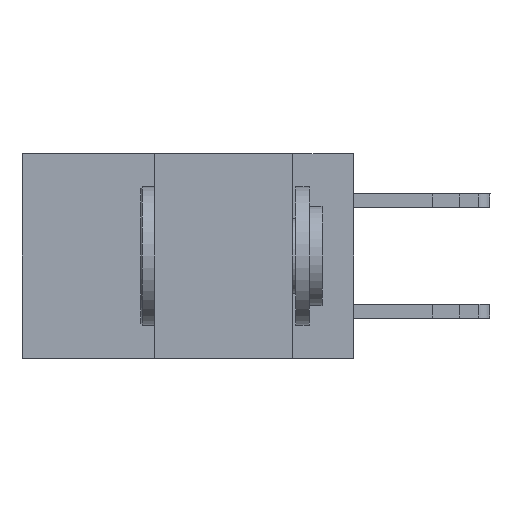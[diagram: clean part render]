
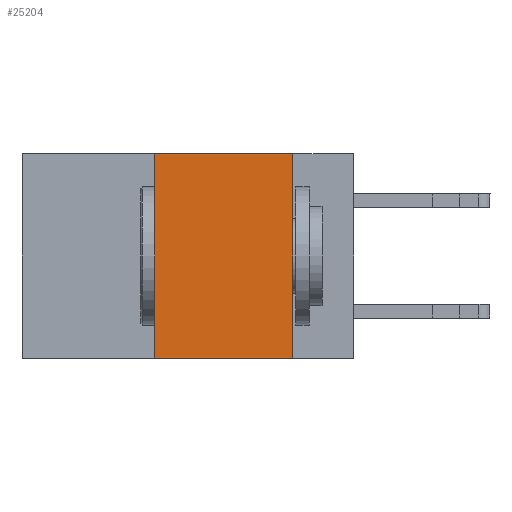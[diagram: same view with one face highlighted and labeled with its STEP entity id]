
A CAD part, left-side view. The second image highlights one B-rep face of the part: STEP entity #25204.
In plain terms, the highlighted planar face has unit normal (-1, 0, 0).
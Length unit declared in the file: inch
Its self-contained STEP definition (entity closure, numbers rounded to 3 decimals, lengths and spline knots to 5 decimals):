
#544 = DIRECTION ( 'NONE',  ( 0., -1., 0. ) ) ;
#687 = AXIS2_PLACEMENT_3D ( 'NONE', #19493, #21881, #11648 ) ;
#3973 = EDGE_CURVE ( 'NONE', #22926, #3980, #19147, .T. ) ;
#3980 = VERTEX_POINT ( 'NONE', #6710 ) ;
#4710 = VECTOR ( 'NONE', #15154, 39.37008 ) ;
#5445 = FACE_OUTER_BOUND ( 'NONE', #15255, .T. ) ;
#6233 = EDGE_CURVE ( 'NONE', #8198, #3980, #22559, .T. ) ;
#6710 = CARTESIAN_POINT ( 'NONE',  ( 0., 0.11, -0.37 ) ) ;
#7871 = EDGE_CURVE ( 'NONE', #22926, #14827, #20736, .T. ) ;
#8198 = VERTEX_POINT ( 'NONE', #24194 ) ;
#8644 = ORIENTED_EDGE ( 'NONE', *, *, #6233, .F. ) ;
#9062 = CARTESIAN_POINT ( 'NONE',  ( 0., 0.36, 0. ) ) ;
#9498 = VECTOR ( 'NONE', #22444, 39.37008 ) ;
#10310 = CARTESIAN_POINT ( 'NONE',  ( 0., 0.36, -0.37 ) ) ;
#10762 = LINE ( 'NONE', #24233, #25164 ) ;
#11648 = DIRECTION ( 'NONE',  ( 0., 0., -1. ) ) ;
#12267 = VECTOR ( 'NONE', #12719, 39.37008 ) ;
#12635 = CARTESIAN_POINT ( 'NONE',  ( 0., 0.6, -0.37 ) ) ;
#12719 = DIRECTION ( 'NONE',  ( 0., 0., 1. ) ) ;
#13133 = ORIENTED_EDGE ( 'NONE', *, *, #16784, .F. ) ;
#14554 = CARTESIAN_POINT ( 'NONE',  ( 0., 0.36, 0. ) ) ;
#14827 = VERTEX_POINT ( 'NONE', #14554 ) ;
#15154 = DIRECTION ( 'NONE',  ( 0., 0., -1. ) ) ;
#15255 = EDGE_LOOP ( 'NONE', ( #8644, #13133, #18487, #18840 ) ) ;
#15462 = PLANE ( 'NONE',  #687 ) ;
#16107 = CARTESIAN_POINT ( 'NONE',  ( 0., 0.11, 0. ) ) ;
#16784 = EDGE_CURVE ( 'NONE', #14827, #8198, #10762, .T. ) ;
#18487 = ORIENTED_EDGE ( 'NONE', *, *, #7871, .F. ) ;
#18840 = ORIENTED_EDGE ( 'NONE', *, *, #3973, .T. ) ;
#19147 = LINE ( 'NONE', #12635, #9498 ) ;
#19493 = CARTESIAN_POINT ( 'NONE',  ( 0., 0.6, 0. ) ) ;
#20736 = LINE ( 'NONE', #9062, #12267 ) ;
#21881 = DIRECTION ( 'NONE',  ( 1., 0., 0. ) ) ;
#22444 = DIRECTION ( 'NONE',  ( 0., -1., 0. ) ) ;
#22559 = LINE ( 'NONE', #16107, #4710 ) ;
#22926 = VERTEX_POINT ( 'NONE', #10310 ) ;
#24194 = CARTESIAN_POINT ( 'NONE',  ( 0., 0.11, 0. ) ) ;
#24233 = CARTESIAN_POINT ( 'NONE',  ( 0., 0.6, 0. ) ) ;
#25164 = VECTOR ( 'NONE', #544, 39.37008 ) ;
#25204 = ADVANCED_FACE ( 'NONE', ( #5445 ), #15462, .F. ) ;
